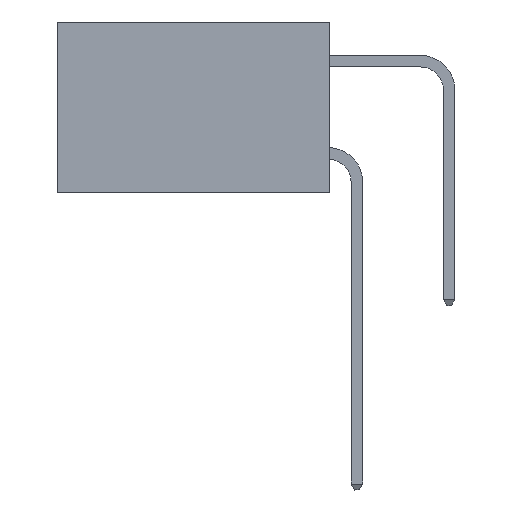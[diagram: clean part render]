
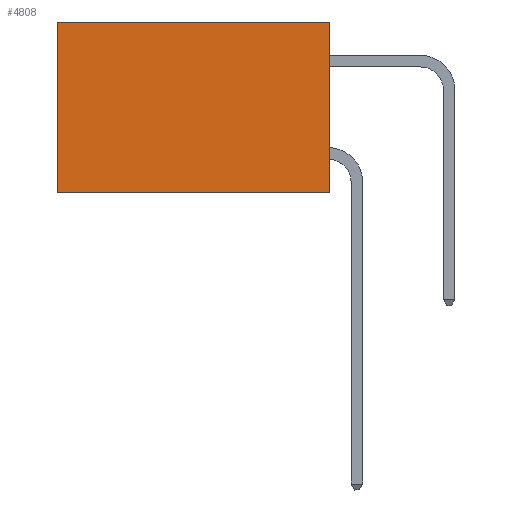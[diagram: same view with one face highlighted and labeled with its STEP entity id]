
A CAD part, left-side view. The second image highlights one B-rep face of the part: STEP entity #4808.
In plain terms, the highlighted planar face has unit normal (-1, 0, 0).
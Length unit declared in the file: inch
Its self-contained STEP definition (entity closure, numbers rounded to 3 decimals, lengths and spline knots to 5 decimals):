
#643 = LINE ( 'NONE', #2236, #3799 ) ;
#1375 = CARTESIAN_POINT ( 'NONE',  ( 0.277, 0., 0. ) ) ;
#1627 = CARTESIAN_POINT ( 'NONE',  ( 0.277, 0.59, 0. ) ) ;
#2031 = DIRECTION ( 'NONE',  ( 0., 0., -1. ) ) ;
#2154 = DIRECTION ( 'NONE',  ( 0., 0., -1. ) ) ;
#2236 = CARTESIAN_POINT ( 'NONE',  ( 0.277, 0., -0.37 ) ) ;
#2548 = EDGE_LOOP ( 'NONE', ( #15431, #17396, #12880, #3075 ) ) ;
#2689 = VERTEX_POINT ( 'NONE', #14939 ) ;
#3075 = ORIENTED_EDGE ( 'NONE', *, *, #14025, .T. ) ;
#3606 = DIRECTION ( 'NONE',  ( 0., 1., 0. ) ) ;
#3799 = VECTOR ( 'NONE', #2154, 39.37008 ) ;
#4808 = ADVANCED_FACE ( 'NONE', ( #6029 ), #7455, .F. ) ;
#5414 = CARTESIAN_POINT ( 'NONE',  ( 0.277, 0., -0.37 ) ) ;
#5560 = DIRECTION ( 'NONE',  ( 0., 1., 0. ) ) ;
#5912 = LINE ( 'NONE', #8209, #13452 ) ;
#6029 = FACE_OUTER_BOUND ( 'NONE', #2548, .T. ) ;
#6810 = EDGE_CURVE ( 'NONE', #12525, #2689, #643, .T. ) ;
#7455 = PLANE ( 'NONE',  #17447 ) ;
#8209 = CARTESIAN_POINT ( 'NONE',  ( 0.277, 0., -0.37 ) ) ;
#8663 = LINE ( 'NONE', #13073, #11215 ) ;
#9565 = CARTESIAN_POINT ( 'NONE',  ( 0.277, 0.59, -0.37 ) ) ;
#10312 = VERTEX_POINT ( 'NONE', #12847 ) ;
#10501 = DIRECTION ( 'NONE',  ( 1., 0., 0. ) ) ;
#10865 = EDGE_CURVE ( 'NONE', #2689, #10312, #5912, .T. ) ;
#11082 = DIRECTION ( 'NONE',  ( 0., 0., -1. ) ) ;
#11215 = VECTOR ( 'NONE', #5560, 39.37008 ) ;
#11360 = EDGE_CURVE ( 'NONE', #15766, #10312, #13431, .T. ) ;
#12525 = VERTEX_POINT ( 'NONE', #1375 ) ;
#12847 = CARTESIAN_POINT ( 'NONE',  ( 0.277, 0.59, -0.37 ) ) ;
#12880 = ORIENTED_EDGE ( 'NONE', *, *, #6810, .F. ) ;
#12954 = VECTOR ( 'NONE', #11082, 39.37008 ) ;
#13073 = CARTESIAN_POINT ( 'NONE',  ( 0.277, 0., 0. ) ) ;
#13431 = LINE ( 'NONE', #9565, #12954 ) ;
#13452 = VECTOR ( 'NONE', #3606, 39.37008 ) ;
#14025 = EDGE_CURVE ( 'NONE', #12525, #15766, #8663, .T. ) ;
#14939 = CARTESIAN_POINT ( 'NONE',  ( 0.277, 0., -0.37 ) ) ;
#15431 = ORIENTED_EDGE ( 'NONE', *, *, #11360, .T. ) ;
#15766 = VERTEX_POINT ( 'NONE', #1627 ) ;
#17396 = ORIENTED_EDGE ( 'NONE', *, *, #10865, .F. ) ;
#17447 = AXIS2_PLACEMENT_3D ( 'NONE', #5414, #10501, #2031 ) ;
